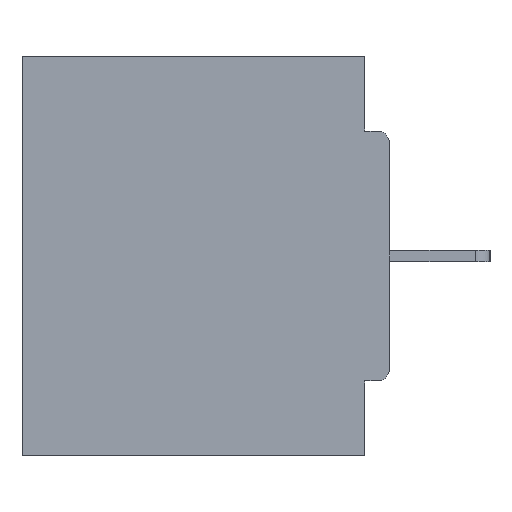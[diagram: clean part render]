
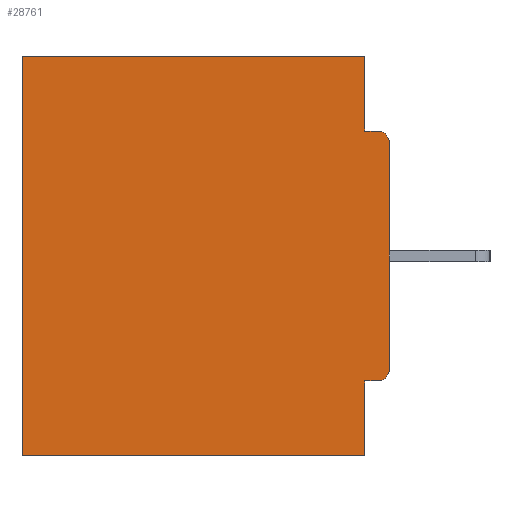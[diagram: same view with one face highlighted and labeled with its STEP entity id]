
A CAD part, left-side view. The second image highlights one B-rep face of the part: STEP entity #28761.
In plain terms, the highlighted planar face has unit normal (-1, 0, 0).
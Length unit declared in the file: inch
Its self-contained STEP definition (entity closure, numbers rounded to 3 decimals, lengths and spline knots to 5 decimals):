
#118 = DIRECTION ( 'NONE',  ( -1., 0., 0. ) ) ;
#543 = DIRECTION ( 'NONE',  ( 0., 0., -1. ) ) ;
#777 = CARTESIAN_POINT ( 'NONE',  ( 0.298, 0.031, -0.0935 ) ) ;
#943 = CARTESIAN_POINT ( 'NONE',  ( 0.298, 0.015, -0.0935 ) ) ;
#1493 = VECTOR ( 'NONE', #24996, 39.37008 ) ;
#1537 = VECTOR ( 'NONE', #16554, 39.37008 ) ;
#1833 = FACE_OUTER_BOUND ( 'NONE', #17816, .T. ) ;
#1866 = VERTEX_POINT ( 'NONE', #7962 ) ;
#2607 = VECTOR ( 'NONE', #2809, 39.37008 ) ;
#2809 = DIRECTION ( 'NONE',  ( 0., 0., -1. ) ) ;
#3066 = VERTEX_POINT ( 'NONE', #943 ) ;
#3375 = VERTEX_POINT ( 'NONE', #13440 ) ;
#3645 = DIRECTION ( 'NONE',  ( 0., 0., -1. ) ) ;
#3824 = EDGE_CURVE ( 'NONE', #14580, #4561, #9539, .T. ) ;
#4561 = VERTEX_POINT ( 'NONE', #14929 ) ;
#4574 = LINE ( 'NONE', #13425, #1493 ) ;
#5023 = CARTESIAN_POINT ( 'NONE',  ( 0.298, 0., -0.5 ) ) ;
#5145 = ORIENTED_EDGE ( 'NONE', *, *, #25105, .T. ) ;
#5322 = EDGE_CURVE ( 'NONE', #14580, #25049, #17243, .T. ) ;
#5876 = ORIENTED_EDGE ( 'NONE', *, *, #3824, .T. ) ;
#6326 = EDGE_CURVE ( 'NONE', #26178, #23997, #17765, .T. ) ;
#6409 = CARTESIAN_POINT ( 'NONE',  ( 0.298, 0., 0. ) ) ;
#6645 = VERTEX_POINT ( 'NONE', #777 ) ;
#7065 = LINE ( 'NONE', #11479, #2607 ) ;
#7223 = ORIENTED_EDGE ( 'NONE', *, *, #25688, .F. ) ;
#7799 = ORIENTED_EDGE ( 'NONE', *, *, #5322, .F. ) ;
#7962 = CARTESIAN_POINT ( 'NONE',  ( 0.298, 0., -0.1085 ) ) ;
#8055 = CARTESIAN_POINT ( 'NONE',  ( 0.298, 0.015, -0.1085 ) ) ;
#8182 = ORIENTED_EDGE ( 'NONE', *, *, #12223, .F. ) ;
#8330 = LINE ( 'NONE', #6409, #22888 ) ;
#8605 = DIRECTION ( 'NONE',  ( 0., 0., -1. ) ) ;
#9448 = LINE ( 'NONE', #5023, #15245 ) ;
#9539 = CIRCLE ( 'NONE', #27076, 0.015 ) ;
#9815 = AXIS2_PLACEMENT_3D ( 'NONE', #13164, #19843, #8605 ) ;
#10144 = VECTOR ( 'NONE', #13300, 39.37008 ) ;
#10403 = VECTOR ( 'NONE', #24321, 39.37008 ) ;
#11217 = LINE ( 'NONE', #13149, #10144 ) ;
#11479 = CARTESIAN_POINT ( 'NONE',  ( 0.298, 0., 0. ) ) ;
#11810 = EDGE_CURVE ( 'NONE', #25049, #23604, #4574, .T. ) ;
#12223 = EDGE_CURVE ( 'NONE', #6645, #3066, #23140, .T. ) ;
#12726 = CARTESIAN_POINT ( 'NONE',  ( 0.298, 0.46, 0. ) ) ;
#12847 = CARTESIAN_POINT ( 'NONE',  ( 0.298, 0.031, -0.5 ) ) ;
#13149 = CARTESIAN_POINT ( 'NONE',  ( 0.298, 0.031, -0.5 ) ) ;
#13164 = CARTESIAN_POINT ( 'NONE',  ( 0.298, 0., 0. ) ) ;
#13300 = DIRECTION ( 'NONE',  ( 0., 0., -1. ) ) ;
#13425 = CARTESIAN_POINT ( 'NONE',  ( 0.298, 0.031, -0.5 ) ) ;
#13431 = AXIS2_PLACEMENT_3D ( 'NONE', #8055, #24358, #3645 ) ;
#13440 = CARTESIAN_POINT ( 'NONE',  ( 0.298, 0.031, 0. ) ) ;
#14580 = VERTEX_POINT ( 'NONE', #28475 ) ;
#14667 = EDGE_CURVE ( 'NONE', #3375, #26178, #8330, .T. ) ;
#14697 = CARTESIAN_POINT ( 'NONE',  ( 0.298, 0.031, -0.4065 ) ) ;
#14929 = CARTESIAN_POINT ( 'NONE',  ( 0.298, 0., -0.3915 ) ) ;
#15245 = VECTOR ( 'NONE', #23101, 39.37008 ) ;
#15386 = PLANE ( 'NONE',  #9815 ) ;
#15403 = DIRECTION ( 'NONE',  ( 0., 1., 0. ) ) ;
#15852 = ORIENTED_EDGE ( 'NONE', *, *, #22400, .F. ) ;
#16554 = DIRECTION ( 'NONE',  ( 0., 1., 0. ) ) ;
#16823 = EDGE_CURVE ( 'NONE', #1866, #4561, #7065, .T. ) ;
#17243 = LINE ( 'NONE', #27528, #1537 ) ;
#17765 = LINE ( 'NONE', #12726, #10403 ) ;
#17816 = EDGE_LOOP ( 'NONE', ( #5145, #8182, #7223, #26414, #23720, #15852, #27560, #7799, #5876, #22648 ) ) ;
#18678 = CARTESIAN_POINT ( 'NONE',  ( 0.298, 0., -0.0935 ) ) ;
#19406 = VECTOR ( 'NONE', #27721, 39.37008 ) ;
#19843 = DIRECTION ( 'NONE',  ( 1., 0., 0. ) ) ;
#22400 = EDGE_CURVE ( 'NONE', #23604, #23997, #9448, .T. ) ;
#22648 = ORIENTED_EDGE ( 'NONE', *, *, #16823, .F. ) ;
#22888 = VECTOR ( 'NONE', #15403, 39.37008 ) ;
#23101 = DIRECTION ( 'NONE',  ( 0., 1., 0. ) ) ;
#23140 = LINE ( 'NONE', #18678, #19406 ) ;
#23604 = VERTEX_POINT ( 'NONE', #12847 ) ;
#23720 = ORIENTED_EDGE ( 'NONE', *, *, #6326, .T. ) ;
#23975 = CARTESIAN_POINT ( 'NONE',  ( 0.298, 0.46, -0.5 ) ) ;
#23997 = VERTEX_POINT ( 'NONE', #23975 ) ;
#24321 = DIRECTION ( 'NONE',  ( 0., 0., -1. ) ) ;
#24358 = DIRECTION ( 'NONE',  ( -1., 0., 0. ) ) ;
#24996 = DIRECTION ( 'NONE',  ( 0., 0., -1. ) ) ;
#25049 = VERTEX_POINT ( 'NONE', #14697 ) ;
#25105 = EDGE_CURVE ( 'NONE', #1866, #3066, #27634, .T. ) ;
#25688 = EDGE_CURVE ( 'NONE', #3375, #6645, #11217, .T. ) ;
#26178 = VERTEX_POINT ( 'NONE', #28993 ) ;
#26414 = ORIENTED_EDGE ( 'NONE', *, *, #14667, .T. ) ;
#27076 = AXIS2_PLACEMENT_3D ( 'NONE', #27299, #118, #543 ) ;
#27299 = CARTESIAN_POINT ( 'NONE',  ( 0.298, 0.015, -0.3915 ) ) ;
#27528 = CARTESIAN_POINT ( 'NONE',  ( 0.298, 0., -0.4065 ) ) ;
#27560 = ORIENTED_EDGE ( 'NONE', *, *, #11810, .F. ) ;
#27634 = CIRCLE ( 'NONE', #13431, 0.015 ) ;
#27721 = DIRECTION ( 'NONE',  ( 0., -1., 0. ) ) ;
#28475 = CARTESIAN_POINT ( 'NONE',  ( 0.298, 0.015, -0.4065 ) ) ;
#28761 = ADVANCED_FACE ( 'NONE', ( #1833 ), #15386, .F. ) ;
#28993 = CARTESIAN_POINT ( 'NONE',  ( 0.298, 0.46, 0. ) ) ;
